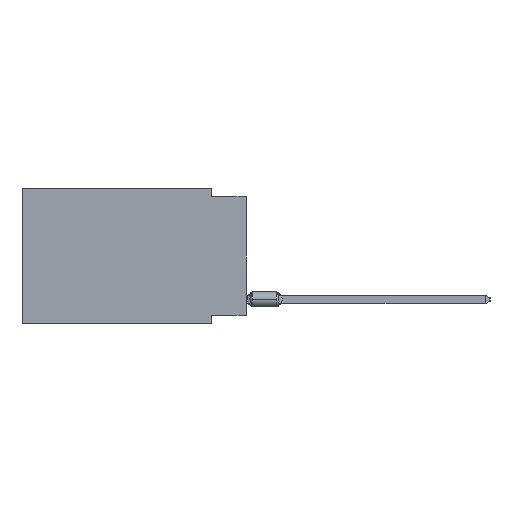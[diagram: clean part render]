
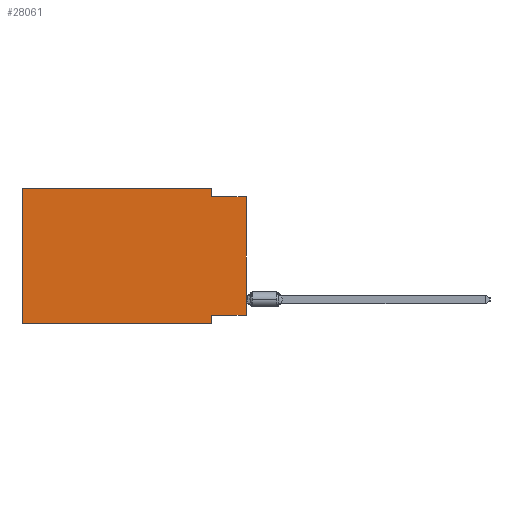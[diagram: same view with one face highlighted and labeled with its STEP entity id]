
A CAD part, left-side view. The second image highlights one B-rep face of the part: STEP entity #28061.
In plain terms, the highlighted planar face has unit normal (-1, 0, 0).
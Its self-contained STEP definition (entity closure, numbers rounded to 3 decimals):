
#112 = AXIS2_PLACEMENT_3D ( 'NONE', #14230, #28787, #14411 ) ;
#127 = CARTESIAN_POINT ( 'NONE',  ( 0., 2.54, 0. ) ) ;
#305 = CARTESIAN_POINT ( 'NONE',  ( 0., 16.383, 0. ) ) ;
#798 = CARTESIAN_POINT ( 'NONE',  ( 0., 2.54, -9.271 ) ) ;
#913 = CARTESIAN_POINT ( 'NONE',  ( 0., 2.54, -9.906 ) ) ;
#1024 = ORIENTED_EDGE ( 'NONE', *, *, #7748, .F. ) ;
#1845 = LINE ( 'NONE', #27642, #20085 ) ;
#2049 = DIRECTION ( 'NONE',  ( 0., 0., 1. ) ) ;
#2789 = CARTESIAN_POINT ( 'NONE',  ( 0., 16.383, 0. ) ) ;
#2832 = FACE_OUTER_BOUND ( 'NONE', #6990, .T. ) ;
#2904 = VERTEX_POINT ( 'NONE', #2789 ) ;
#3130 = ORIENTED_EDGE ( 'NONE', *, *, #22730, .F. ) ;
#3279 = LINE ( 'NONE', #4039, #27333 ) ;
#4039 = CARTESIAN_POINT ( 'NONE',  ( 0., 0., -0.635 ) ) ;
#5564 = CARTESIAN_POINT ( 'NONE',  ( 0., 2.54, 0. ) ) ;
#6034 = EDGE_CURVE ( 'NONE', #24824, #11010, #8399, .T. ) ;
#6990 = EDGE_LOOP ( 'NONE', ( #24621, #3130, #35415, #1024, #31169, #17294, #29882, #9376 ) ) ;
#7748 = EDGE_CURVE ( 'NONE', #2904, #33441, #9213, .T. ) ;
#8399 = LINE ( 'NONE', #26007, #13153 ) ;
#8688 = DIRECTION ( 'NONE',  ( 0., 0., -1. ) ) ;
#9213 = LINE ( 'NONE', #305, #27644 ) ;
#9376 = ORIENTED_EDGE ( 'NONE', *, *, #35104, .F. ) ;
#11010 = VERTEX_POINT ( 'NONE', #31186 ) ;
#11699 = VERTEX_POINT ( 'NONE', #37337 ) ;
#11743 = CARTESIAN_POINT ( 'NONE',  ( 0., 0., -0.635 ) ) ;
#11900 = DIRECTION ( 'NONE',  ( 0., -1., 0. ) ) ;
#13153 = VECTOR ( 'NONE', #31679, 1000. ) ;
#14230 = CARTESIAN_POINT ( 'NONE',  ( 0., 16.383, 0. ) ) ;
#14411 = DIRECTION ( 'NONE',  ( 0., 0., -1. ) ) ;
#15213 = LINE ( 'NONE', #32429, #15396 ) ;
#15329 = DIRECTION ( 'NONE',  ( 0., 0., -1. ) ) ;
#15396 = VECTOR ( 'NONE', #26745, 1000. ) ;
#16770 = VERTEX_POINT ( 'NONE', #11743 ) ;
#17265 = PLANE ( 'NONE',  #112 ) ;
#17294 = ORIENTED_EDGE ( 'NONE', *, *, #6034, .T. ) ;
#17354 = CARTESIAN_POINT ( 'NONE',  ( 0., 0., -9.271 ) ) ;
#20035 = CARTESIAN_POINT ( 'NONE',  ( 0., 0., -9.271 ) ) ;
#20085 = VECTOR ( 'NONE', #2049, 1000. ) ;
#20730 = DIRECTION ( 'NONE',  ( 0., 1., 0. ) ) ;
#22730 = EDGE_CURVE ( 'NONE', #11699, #16770, #3279, .T. ) ;
#23317 = VECTOR ( 'NONE', #20730, 1000. ) ;
#23509 = EDGE_CURVE ( 'NONE', #33441, #11699, #28944, .T. ) ;
#23950 = DIRECTION ( 'NONE',  ( 0., -1., 0. ) ) ;
#24621 = ORIENTED_EDGE ( 'NONE', *, *, #25079, .T. ) ;
#24824 = VERTEX_POINT ( 'NONE', #36399 ) ;
#25079 = EDGE_CURVE ( 'NONE', #32951, #16770, #15213, .T. ) ;
#26007 = CARTESIAN_POINT ( 'NONE',  ( 0., 16.383, -9.906 ) ) ;
#26168 = VECTOR ( 'NONE', #8688, 1000. ) ;
#26745 = DIRECTION ( 'NONE',  ( 0., 0., 1. ) ) ;
#27333 = VECTOR ( 'NONE', #23950, 1000. ) ;
#27642 = CARTESIAN_POINT ( 'NONE',  ( 0., 16.383, 0. ) ) ;
#27644 = VECTOR ( 'NONE', #11900, 1000. ) ;
#28061 = ADVANCED_FACE ( 'NONE', ( #2832 ), #17265, .F. ) ;
#28787 = DIRECTION ( 'NONE',  ( 1., 0., 0. ) ) ;
#28944 = LINE ( 'NONE', #127, #26168 ) ;
#29882 = ORIENTED_EDGE ( 'NONE', *, *, #34409, .F. ) ;
#30875 = VERTEX_POINT ( 'NONE', #798 ) ;
#31169 = ORIENTED_EDGE ( 'NONE', *, *, #31365, .F. ) ;
#31186 = CARTESIAN_POINT ( 'NONE',  ( 0., 2.54, -9.906 ) ) ;
#31365 = EDGE_CURVE ( 'NONE', #24824, #2904, #1845, .T. ) ;
#31679 = DIRECTION ( 'NONE',  ( 0., -1., 0. ) ) ;
#32142 = LINE ( 'NONE', #913, #34143 ) ;
#32429 = CARTESIAN_POINT ( 'NONE',  ( 0., 0., 0. ) ) ;
#32951 = VERTEX_POINT ( 'NONE', #20035 ) ;
#33441 = VERTEX_POINT ( 'NONE', #5564 ) ;
#34143 = VECTOR ( 'NONE', #15329, 1000. ) ;
#34409 = EDGE_CURVE ( 'NONE', #30875, #11010, #32142, .T. ) ;
#35104 = EDGE_CURVE ( 'NONE', #32951, #30875, #37362, .T. ) ;
#35415 = ORIENTED_EDGE ( 'NONE', *, *, #23509, .F. ) ;
#36399 = CARTESIAN_POINT ( 'NONE',  ( 0., 16.383, -9.906 ) ) ;
#37337 = CARTESIAN_POINT ( 'NONE',  ( 0., 2.54, -0.635 ) ) ;
#37362 = LINE ( 'NONE', #17354, #23317 ) ;
